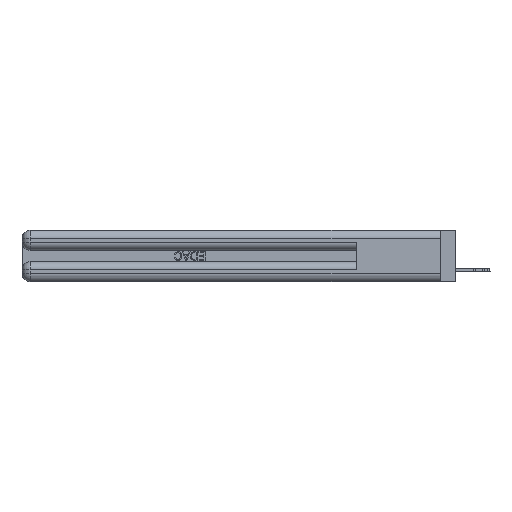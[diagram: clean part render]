
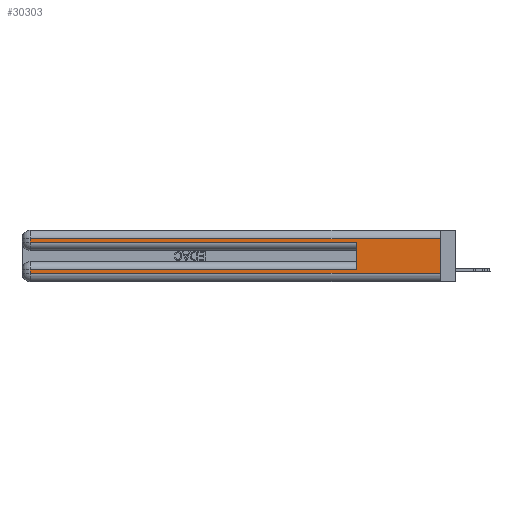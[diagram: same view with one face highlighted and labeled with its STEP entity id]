
A CAD part, left-side view. The second image highlights one B-rep face of the part: STEP entity #30303.
In plain terms, the highlighted planar face has unit normal (-1, 0, 0).
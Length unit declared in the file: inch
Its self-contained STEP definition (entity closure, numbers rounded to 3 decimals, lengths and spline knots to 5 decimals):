
#623 = AXIS2_PLACEMENT_3D ( 'NONE', #35715, #25107, #873 ) ;
#698 = CARTESIAN_POINT ( 'NONE',  ( 0., 0., 0.31 ) ) ;
#836 = VERTEX_POINT ( 'NONE', #28149 ) ;
#873 = DIRECTION ( 'NONE',  ( 0., 0., -1. ) ) ;
#1037 = LINE ( 'NONE', #37953, #16823 ) ;
#1326 = ORIENTED_EDGE ( 'NONE', *, *, #39877, .T. ) ;
#2086 = VECTOR ( 'NONE', #14432, 39.37008 ) ;
#3133 = VERTEX_POINT ( 'NONE', #34230 ) ;
#3198 = CARTESIAN_POINT ( 'NONE',  ( 0., 0., 0.085 ) ) ;
#5669 = EDGE_CURVE ( 'NONE', #836, #3133, #35351, .T. ) ;
#5861 = DIRECTION ( 'NONE',  ( 0., 1., 0. ) ) ;
#7338 = EDGE_CURVE ( 'NONE', #36405, #31468, #30278, .T. ) ;
#8318 = DIRECTION ( 'NONE',  ( 0., -1., 0. ) ) ;
#8506 = VECTOR ( 'NONE', #37464, 39.37008 ) ;
#8632 = EDGE_CURVE ( 'NONE', #836, #31468, #37874, .T. ) ;
#9582 = EDGE_CURVE ( 'NONE', #21156, #36405, #30163, .T. ) ;
#10254 = DIRECTION ( 'NONE',  ( 0., 0., -1. ) ) ;
#10433 = EDGE_CURVE ( 'NONE', #26337, #13639, #22066, .T. ) ;
#10991 = LINE ( 'NONE', #33651, #34299 ) ;
#12259 = LINE ( 'NONE', #16061, #8506 ) ;
#13639 = VERTEX_POINT ( 'NONE', #31774 ) ;
#14432 = DIRECTION ( 'NONE',  ( 0., 0., 1. ) ) ;
#15771 = DIRECTION ( 'NONE',  ( 0., 0., -1. ) ) ;
#16061 = CARTESIAN_POINT ( 'NONE',  ( 0., 0., 0.37 ) ) ;
#16266 = VERTEX_POINT ( 'NONE', #698 ) ;
#16823 = VECTOR ( 'NONE', #10254, 39.37008 ) ;
#17250 = CARTESIAN_POINT ( 'NONE',  ( 0., 0., 0.285 ) ) ;
#18953 = ORIENTED_EDGE ( 'NONE', *, *, #20889, .T. ) ;
#18970 = CARTESIAN_POINT ( 'NONE',  ( 0., 2.94, 0.37 ) ) ;
#20475 = ORIENTED_EDGE ( 'NONE', *, *, #9582, .T. ) ;
#20560 = DIRECTION ( 'NONE',  ( 0., 1., 0. ) ) ;
#20889 = EDGE_CURVE ( 'NONE', #3133, #26337, #1037, .T. ) ;
#21156 = VERTEX_POINT ( 'NONE', #33650 ) ;
#21634 = ORIENTED_EDGE ( 'NONE', *, *, #7338, .T. ) ;
#22066 = LINE ( 'NONE', #29003, #43814 ) ;
#22106 = ORIENTED_EDGE ( 'NONE', *, *, #5669, .T. ) ;
#23218 = CARTESIAN_POINT ( 'NONE',  ( 0., 0.6, 0.285 ) ) ;
#24708 = CARTESIAN_POINT ( 'NONE',  ( 0., 2.94, 0.06 ) ) ;
#25069 = ORIENTED_EDGE ( 'NONE', *, *, #8632, .F. ) ;
#25107 = DIRECTION ( 'NONE',  ( 1., 0., 0. ) ) ;
#25286 = VECTOR ( 'NONE', #15771, 39.37008 ) ;
#26337 = VERTEX_POINT ( 'NONE', #24708 ) ;
#27670 = ORIENTED_EDGE ( 'NONE', *, *, #43742, .F. ) ;
#28149 = CARTESIAN_POINT ( 'NONE',  ( 0., 0.6, 0.085 ) ) ;
#28302 = VECTOR ( 'NONE', #20560, 39.37008 ) ;
#29003 = CARTESIAN_POINT ( 'NONE',  ( 0., 0., 0.06 ) ) ;
#30163 = LINE ( 'NONE', #18970, #25286 ) ;
#30278 = LINE ( 'NONE', #17250, #37939 ) ;
#30303 = ADVANCED_FACE ( 'NONE', ( #37599 ), #35556, .F. ) ;
#31468 = VERTEX_POINT ( 'NONE', #23218 ) ;
#31774 = CARTESIAN_POINT ( 'NONE',  ( 0., 0., 0.06 ) ) ;
#33650 = CARTESIAN_POINT ( 'NONE',  ( 0., 2.94, 0.31 ) ) ;
#33651 = CARTESIAN_POINT ( 'NONE',  ( 0., 0., 0.31 ) ) ;
#34230 = CARTESIAN_POINT ( 'NONE',  ( 0., 2.94, 0.085 ) ) ;
#34299 = VECTOR ( 'NONE', #5861, 39.37008 ) ;
#35351 = LINE ( 'NONE', #3198, #28302 ) ;
#35556 = PLANE ( 'NONE',  #623 ) ;
#35715 = CARTESIAN_POINT ( 'NONE',  ( 0., 0., 0.37 ) ) ;
#36405 = VERTEX_POINT ( 'NONE', #42776 ) ;
#37125 = EDGE_LOOP ( 'NONE', ( #27670, #1326, #20475, #21634, #25069, #22106, #18953, #44574 ) ) ;
#37464 = DIRECTION ( 'NONE',  ( 0., 0., -1. ) ) ;
#37599 = FACE_OUTER_BOUND ( 'NONE', #37125, .T. ) ;
#37815 = CARTESIAN_POINT ( 'NONE',  ( 0., 0.6, 0.145 ) ) ;
#37874 = LINE ( 'NONE', #37815, #2086 ) ;
#37939 = VECTOR ( 'NONE', #38296, 39.37008 ) ;
#37953 = CARTESIAN_POINT ( 'NONE',  ( 0., 2.94, 0.37 ) ) ;
#38296 = DIRECTION ( 'NONE',  ( 0., -1., 0. ) ) ;
#39877 = EDGE_CURVE ( 'NONE', #16266, #21156, #10991, .T. ) ;
#42776 = CARTESIAN_POINT ( 'NONE',  ( 0., 2.94, 0.285 ) ) ;
#43742 = EDGE_CURVE ( 'NONE', #16266, #13639, #12259, .T. ) ;
#43814 = VECTOR ( 'NONE', #8318, 39.37008 ) ;
#44574 = ORIENTED_EDGE ( 'NONE', *, *, #10433, .T. ) ;
